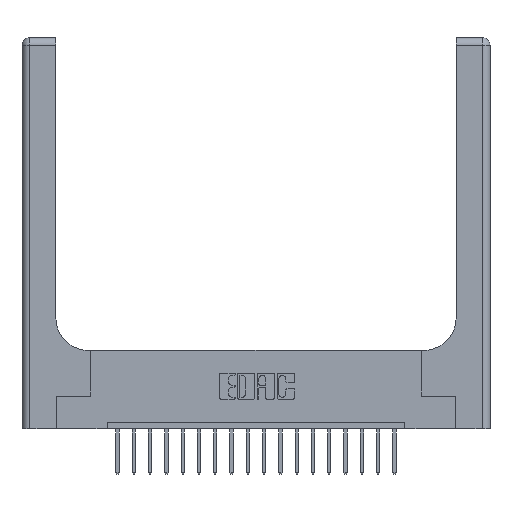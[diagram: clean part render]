
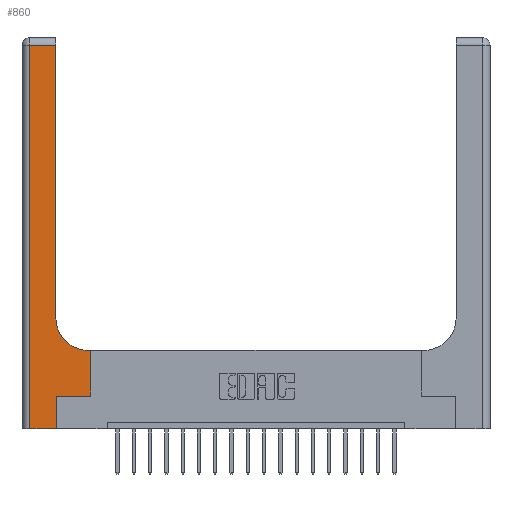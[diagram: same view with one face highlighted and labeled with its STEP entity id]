
A CAD part, top view. The second image highlights one B-rep face of the part: STEP entity #860.
In plain terms, the highlighted planar face has unit normal (0, 0, 1).
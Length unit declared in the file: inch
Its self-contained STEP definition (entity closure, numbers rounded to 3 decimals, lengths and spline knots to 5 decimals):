
#37 = CARTESIAN_POINT ( 'NONE',  ( 0.528, 0.25, 0.37 ) ) ;
#201 = VECTOR ( 'NONE', #17152, 39.37008 ) ;
#251 = CARTESIAN_POINT ( 'NONE',  ( 0.26, 2.94, 0.37 ) ) ;
#504 = DIRECTION ( 'NONE',  ( 1., 0., 0. ) ) ;
#577 = VERTEX_POINT ( 'NONE', #251 ) ;
#580 = LINE ( 'NONE', #11638, #16017 ) ;
#750 = ORIENTED_EDGE ( 'NONE', *, *, #12543, .T. ) ;
#751 = DIRECTION ( 'NONE',  ( 1., 0., 0. ) ) ;
#860 = ADVANCED_FACE ( 'NONE', ( #18194 ), #3069, .F. ) ;
#898 = DIRECTION ( 'NONE',  ( 0., 1., 0. ) ) ;
#1443 = EDGE_CURVE ( 'NONE', #4057, #8905, #8883, .T. ) ;
#1683 = CARTESIAN_POINT ( 'NONE',  ( 0.51, 0.6, 0.37 ) ) ;
#1753 = DIRECTION ( 'NONE',  ( 0., 1., 0. ) ) ;
#1853 = DIRECTION ( 'NONE',  ( 1., 0., 0. ) ) ;
#2327 = EDGE_CURVE ( 'NONE', #13740, #4057, #19961, .T. ) ;
#2489 = CARTESIAN_POINT ( 'NONE',  ( 0.06, 2.94, 0.37 ) ) ;
#2494 = VECTOR ( 'NONE', #11857, 39.37008 ) ;
#2521 = ORIENTED_EDGE ( 'NONE', *, *, #1443, .T. ) ;
#3069 = PLANE ( 'NONE',  #10522 ) ;
#3318 = VECTOR ( 'NONE', #1753, 39.37008 ) ;
#3374 = VECTOR ( 'NONE', #1853, 39.37008 ) ;
#3650 = CARTESIAN_POINT ( 'NONE',  ( 0.26, 0.85, 0.37 ) ) ;
#3772 = DIRECTION ( 'NONE',  ( 0., 1., 0. ) ) ;
#3777 = EDGE_LOOP ( 'NONE', ( #18675, #13517, #19435, #6040, #750, #6518, #12185, #18432, #2521 ) ) ;
#4057 = VERTEX_POINT ( 'NONE', #1683 ) ;
#4572 = DIRECTION ( 'NONE',  ( 0., 0., -1. ) ) ;
#4680 = VERTEX_POINT ( 'NONE', #19406 ) ;
#4969 = CARTESIAN_POINT ( 'NONE',  ( 0.06, 3., 0.37 ) ) ;
#5201 = VECTOR ( 'NONE', #751, 39.37008 ) ;
#5290 = LINE ( 'NONE', #6600, #3318 ) ;
#5651 = LINE ( 'NONE', #11556, #15567 ) ;
#5744 = VERTEX_POINT ( 'NONE', #2489 ) ;
#5834 = EDGE_CURVE ( 'NONE', #8905, #577, #8219, .T. ) ;
#5963 = AXIS2_PLACEMENT_3D ( 'NONE', #17549, #8588, #504 ) ;
#6040 = ORIENTED_EDGE ( 'NONE', *, *, #19104, .T. ) ;
#6518 = ORIENTED_EDGE ( 'NONE', *, *, #13317, .T. ) ;
#6600 = CARTESIAN_POINT ( 'NONE',  ( 0.528, 0.25, 0.37 ) ) ;
#6744 = DIRECTION ( 'NONE',  ( -1., 0., 0. ) ) ;
#7487 = EDGE_CURVE ( 'NONE', #5744, #4680, #10962, .T. ) ;
#8219 = LINE ( 'NONE', #16260, #13270 ) ;
#8335 = LINE ( 'NONE', #17800, #5201 ) ;
#8588 = DIRECTION ( 'NONE',  ( 0., 0., -1. ) ) ;
#8883 = CIRCLE ( 'NONE', #5963, 0.25 ) ;
#8905 = VERTEX_POINT ( 'NONE', #3650 ) ;
#10046 = CARTESIAN_POINT ( 'NONE',  ( 0., 0., 0.37 ) ) ;
#10522 = AXIS2_PLACEMENT_3D ( 'NONE', #12187, #4572, #16576 ) ;
#10962 = LINE ( 'NONE', #4969, #201 ) ;
#11556 = CARTESIAN_POINT ( 'NONE',  ( 0.265, 0., 0.37 ) ) ;
#11638 = CARTESIAN_POINT ( 'NONE',  ( 0., 2.94, 0.37 ) ) ;
#11857 = DIRECTION ( 'NONE',  ( -1., 0., 0. ) ) ;
#12185 = ORIENTED_EDGE ( 'NONE', *, *, #16558, .T. ) ;
#12187 = CARTESIAN_POINT ( 'NONE',  ( 0., 3., 0.37 ) ) ;
#12543 = EDGE_CURVE ( 'NONE', #18283, #16709, #5651, .T. ) ;
#13270 = VECTOR ( 'NONE', #3772, 39.37008 ) ;
#13317 = EDGE_CURVE ( 'NONE', #16709, #17535, #8335, .T. ) ;
#13517 = ORIENTED_EDGE ( 'NONE', *, *, #18249, .T. ) ;
#13740 = VERTEX_POINT ( 'NONE', #17368 ) ;
#14229 = LINE ( 'NONE', #10046, #3374 ) ;
#14983 = CARTESIAN_POINT ( 'NONE',  ( 0.265, 0., 0.37 ) ) ;
#15010 = CARTESIAN_POINT ( 'NONE',  ( 0.26, 0.6, 0.37 ) ) ;
#15567 = VECTOR ( 'NONE', #898, 39.37008 ) ;
#16017 = VECTOR ( 'NONE', #6744, 39.37008 ) ;
#16260 = CARTESIAN_POINT ( 'NONE',  ( 0.26, 3., 0.37 ) ) ;
#16558 = EDGE_CURVE ( 'NONE', #17535, #13740, #5290, .T. ) ;
#16576 = DIRECTION ( 'NONE',  ( -1., 0., 0. ) ) ;
#16709 = VERTEX_POINT ( 'NONE', #19600 ) ;
#17152 = DIRECTION ( 'NONE',  ( 0., -1., 0. ) ) ;
#17368 = CARTESIAN_POINT ( 'NONE',  ( 0.528, 0.6, 0.37 ) ) ;
#17535 = VERTEX_POINT ( 'NONE', #37 ) ;
#17549 = CARTESIAN_POINT ( 'NONE',  ( 0.51, 0.85, 0.37 ) ) ;
#17800 = CARTESIAN_POINT ( 'NONE',  ( 0.265, 0.25, 0.37 ) ) ;
#18194 = FACE_OUTER_BOUND ( 'NONE', #3777, .T. ) ;
#18249 = EDGE_CURVE ( 'NONE', #577, #5744, #580, .T. ) ;
#18283 = VERTEX_POINT ( 'NONE', #14983 ) ;
#18432 = ORIENTED_EDGE ( 'NONE', *, *, #2327, .T. ) ;
#18675 = ORIENTED_EDGE ( 'NONE', *, *, #5834, .T. ) ;
#19104 = EDGE_CURVE ( 'NONE', #4680, #18283, #14229, .T. ) ;
#19406 = CARTESIAN_POINT ( 'NONE',  ( 0.06, 0., 0.37 ) ) ;
#19435 = ORIENTED_EDGE ( 'NONE', *, *, #7487, .T. ) ;
#19600 = CARTESIAN_POINT ( 'NONE',  ( 0.265, 0.25, 0.37 ) ) ;
#19961 = LINE ( 'NONE', #15010, #2494 ) ;
